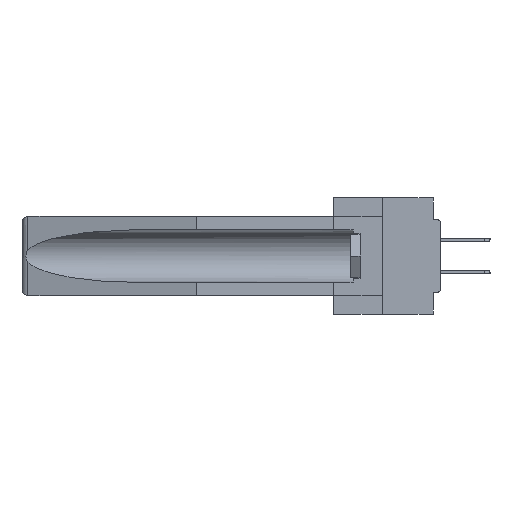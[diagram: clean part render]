
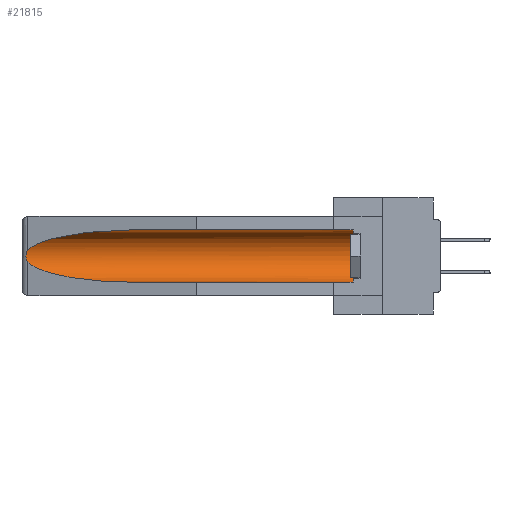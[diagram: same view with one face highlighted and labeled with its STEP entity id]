
A CAD part, left-side view. The second image highlights one B-rep face of the part: STEP entity #21815.
In plain terms, the highlighted cylindrical face has radius 2.857 mm (diameter 5.715 mm), a partial arc.
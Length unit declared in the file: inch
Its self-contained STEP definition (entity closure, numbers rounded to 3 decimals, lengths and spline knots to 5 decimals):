
#3 = CARTESIAN_POINT ( 'NONE',  ( 0.26597, 1.52961, -0.15275 ) ) ;
#1903 = DIRECTION ( 'NONE',  ( 0., 1., 0. ) ) ;
#2954 = EDGE_LOOP ( 'NONE', ( #3526, #16104, #5085, #17953, #12450, #24729 ) ) ;
#3526 = ORIENTED_EDGE ( 'NONE', *, *, #5239, .T. ) ;
#4597 =( BOUNDED_CURVE ( )  B_SPLINE_CURVE ( 3, ( #18400, #6479, #17438, #27581 ),
 .UNSPECIFIED., .F., .T. ) 
 B_SPLINE_CURVE_WITH_KNOTS ( ( 4, 4 ),
 ( 0.1948, 1.5708 ),
 .UNSPECIFIED. ) 
 CURVE ( )  GEOMETRIC_REPRESENTATION_ITEM ( )  RATIONAL_B_SPLINE_CURVE ( ( 1., 0.848, 0.848, 1. ) ) 
 REPRESENTATION_ITEM ( '' )  );
#4640 = CARTESIAN_POINT ( 'NONE',  ( 0.26537, 1.52718, -0.14972 ) ) ;
#5085 = ORIENTED_EDGE ( 'NONE', *, *, #19993, .T. ) ;
#5239 = EDGE_CURVE ( 'NONE', #31595, #38478, #9213, .T. ) ;
#6479 = CARTESIAN_POINT ( 'NONE',  ( 0.25451, 1.48313, -0.24835 ) ) ;
#6602 = EDGE_CURVE ( 'NONE', #38478, #17114, #26876, .T. ) ;
#7779 = DIRECTION ( 'NONE',  ( 0., -1., 0. ) ) ;
#8104 = VERTEX_POINT ( 'NONE', #10673 ) ;
#8896 = CARTESIAN_POINT ( 'NONE',  ( 0.2675, 1.53308, -0.17534 ) ) ;
#9179 = VERTEX_POINT ( 'NONE', #22201 ) ;
#9213 =( BOUNDED_CURVE ( )  B_SPLINE_CURVE ( 3, ( #13246, #28027, #37381, #19349 ),
 .UNSPECIFIED., .F., .F. ) 
 B_SPLINE_CURVE_WITH_KNOTS ( ( 4, 4 ),
 ( 4.71239, 6.08839 ),
 .UNSPECIFIED. ) 
 CURVE ( )  GEOMETRIC_REPRESENTATION_ITEM ( )  RATIONAL_B_SPLINE_CURVE ( ( 1., 0.848, 0.848, 1. ) ) 
 REPRESENTATION_ITEM ( '' )  );
#9270 = CARTESIAN_POINT ( 'NONE',  ( 0.26654, 1.53092, -0.15636 ) ) ;
#9701 = EDGE_CURVE ( 'NONE', #8104, #31595, #17453, .T. ) ;
#10673 = CARTESIAN_POINT ( 'NONE',  ( 0.155, 0.126, -0.059 ) ) ;
#11783 = CARTESIAN_POINT ( 'NONE',  ( 0.2675, 1.53308, -0.16763 ) ) ;
#12450 = ORIENTED_EDGE ( 'NONE', *, *, #24603, .T. ) ;
#13220 = AXIS2_PLACEMENT_3D ( 'NONE', #16901, #7779, #37996 ) ;
#13246 = CARTESIAN_POINT ( 'NONE',  ( 0.155, 1.07973, -0.059 ) ) ;
#13295 = CARTESIAN_POINT ( 'NONE',  ( 0.26537, 1.52718, -0.19328 ) ) ;
#13668 = VECTOR ( 'NONE', #1903, 39.37008 ) ;
#14028 = DIRECTION ( 'NONE',  ( 0., 1., 0. ) ) ;
#14106 = CARTESIAN_POINT ( 'NONE',  ( 0.155, 1.07973, -0.284 ) ) ;
#14148 = LINE ( 'NONE', #32645, #22216 ) ;
#14701 = CARTESIAN_POINT ( 'NONE',  ( 0.26655, 1.53094, -0.18657 ) ) ;
#15098 = CARTESIAN_POINT ( 'NONE',  ( 0.2673, 1.53269, -0.17917 ) ) ;
#16104 = ORIENTED_EDGE ( 'NONE', *, *, #6602, .T. ) ;
#16746 = CYLINDRICAL_SURFACE ( 'NONE', #18761, 0.1125 ) ;
#16844 = CARTESIAN_POINT ( 'NONE',  ( 0.155, -0.30754, -0.059 ) ) ;
#16901 = CARTESIAN_POINT ( 'NONE',  ( 0.155, 0.126, -0.1715 ) ) ;
#17114 = VERTEX_POINT ( 'NONE', #13295 ) ;
#17248 = DIRECTION ( 'NONE',  ( 0., 1., 0. ) ) ;
#17438 = CARTESIAN_POINT ( 'NONE',  ( 0.21114, 1.30732, -0.284 ) ) ;
#17453 = LINE ( 'NONE', #16844, #13668 ) ;
#17681 = CARTESIAN_POINT ( 'NONE',  ( 0.155, 1.07973, -0.059 ) ) ;
#17953 = ORIENTED_EDGE ( 'NONE', *, *, #18303, .F. ) ;
#18303 = EDGE_CURVE ( 'NONE', #9179, #18522, #14148, .T. ) ;
#18400 = CARTESIAN_POINT ( 'NONE',  ( 0.26537, 1.52718, -0.19328 ) ) ;
#18522 = VERTEX_POINT ( 'NONE', #14106 ) ;
#18761 = AXIS2_PLACEMENT_3D ( 'NONE', #19989, #14028, #20502 ) ;
#19349 = CARTESIAN_POINT ( 'NONE',  ( 0.26537, 1.52718, -0.14972 ) ) ;
#19989 = CARTESIAN_POINT ( 'NONE',  ( 0.155, -0.30754, -0.1715 ) ) ;
#19993 = EDGE_CURVE ( 'NONE', #17114, #18522, #4597, .T. ) ;
#20502 = DIRECTION ( 'NONE',  ( 0., 0., 1. ) ) ;
#20925 = CARTESIAN_POINT ( 'NONE',  ( 0.26537, 1.52718, -0.19328 ) ) ;
#21312 = CARTESIAN_POINT ( 'NONE',  ( 0.26537, 1.52718, -0.14972 ) ) ;
#21815 = ADVANCED_FACE ( 'NONE', ( #21961 ), #16746, .F. ) ;
#21961 = FACE_OUTER_BOUND ( 'NONE', #2954, .T. ) ;
#22201 = CARTESIAN_POINT ( 'NONE',  ( 0.155, 0.126, -0.284 ) ) ;
#22216 = VECTOR ( 'NONE', #17248, 39.37008 ) ;
#24603 = EDGE_CURVE ( 'NONE', #9179, #8104, #33955, .T. ) ;
#24729 = ORIENTED_EDGE ( 'NONE', *, *, #9701, .T. ) ;
#26876 = B_SPLINE_CURVE_WITH_KNOTS ( 'NONE', 3,
 ( #21312, #3, #9270, #38857, #11783, #8896, #15098, #14701, #33015, #20925 ),
 .UNSPECIFIED., .F., .F.,
 ( 4, 2, 2, 2, 4 ),
 ( 0., 0.00029, 0.00058, 0.00087, 0.00117 ),
 .UNSPECIFIED. ) ;
#27581 = CARTESIAN_POINT ( 'NONE',  ( 0.155, 1.07973, -0.284 ) ) ;
#28027 = CARTESIAN_POINT ( 'NONE',  ( 0.21114, 1.30732, -0.059 ) ) ;
#31595 = VERTEX_POINT ( 'NONE', #17681 ) ;
#32645 = CARTESIAN_POINT ( 'NONE',  ( 0.155, -0.30754, -0.284 ) ) ;
#33015 = CARTESIAN_POINT ( 'NONE',  ( 0.26597, 1.5296, -0.19026 ) ) ;
#33955 = CIRCLE ( 'NONE', #13220, 0.1125 ) ;
#37381 = CARTESIAN_POINT ( 'NONE',  ( 0.25451, 1.48313, -0.09465 ) ) ;
#37996 = DIRECTION ( 'NONE',  ( 0., 0., 1. ) ) ;
#38478 = VERTEX_POINT ( 'NONE', #4640 ) ;
#38857 = CARTESIAN_POINT ( 'NONE',  ( 0.2673, 1.5327, -0.16383 ) ) ;
